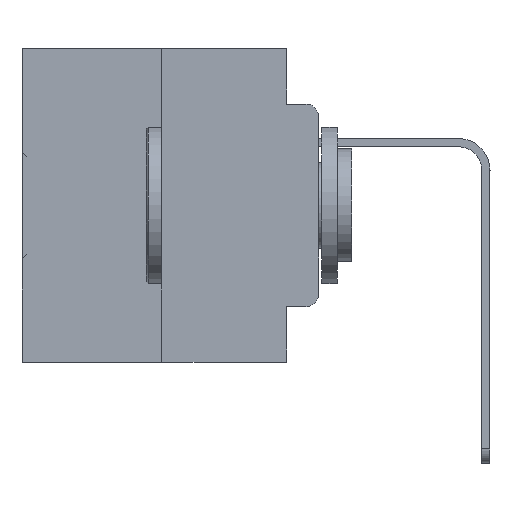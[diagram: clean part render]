
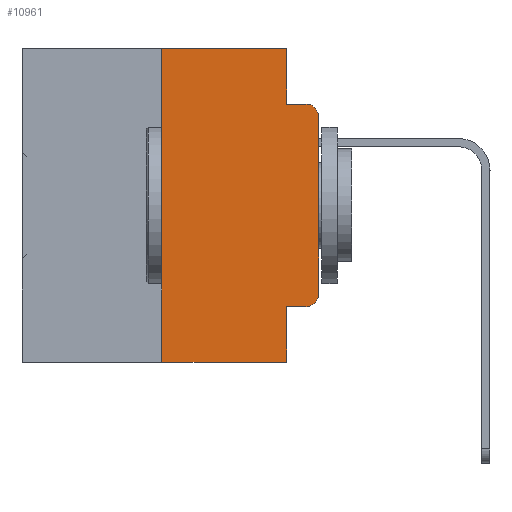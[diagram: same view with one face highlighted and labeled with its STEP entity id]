
A CAD part, left-side view. The second image highlights one B-rep face of the part: STEP entity #10961.
In plain terms, the highlighted planar face has unit normal (-1, 0, 0).
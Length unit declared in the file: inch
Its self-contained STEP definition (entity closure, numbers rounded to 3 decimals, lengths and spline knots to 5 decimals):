
#438 = VERTEX_POINT ( 'NONE', #14731 ) ;
#666 = CARTESIAN_POINT ( 'NONE',  ( 0., 0.051, 0. ) ) ;
#1281 = VERTEX_POINT ( 'NONE', #26488 ) ;
#1385 = CARTESIAN_POINT ( 'NONE',  ( 0., 0., -0.3915 ) ) ;
#1477 = ORIENTED_EDGE ( 'NONE', *, *, #6931, .F. ) ;
#1516 = CARTESIAN_POINT ( 'NONE',  ( 0., 0.473, 0. ) ) ;
#1558 = VERTEX_POINT ( 'NONE', #2695 ) ;
#1998 = DIRECTION ( 'NONE',  ( -1., 0., 0. ) ) ;
#2036 = EDGE_CURVE ( 'NONE', #438, #9720, #26792, .T. ) ;
#2336 = EDGE_CURVE ( 'NONE', #17228, #1281, #18663, .T. ) ;
#2695 = CARTESIAN_POINT ( 'NONE',  ( 0., 0.051, -0.5 ) ) ;
#2988 = CARTESIAN_POINT ( 'NONE',  ( 0., 0.25, 0. ) ) ;
#3020 = ORIENTED_EDGE ( 'NONE', *, *, #28326, .F. ) ;
#4269 = VECTOR ( 'NONE', #19569, 39.37008 ) ;
#4581 = DIRECTION ( 'NONE',  ( 0., 0., -1. ) ) ;
#4801 = EDGE_CURVE ( 'NONE', #17228, #1558, #6444, .T. ) ;
#4955 = VECTOR ( 'NONE', #26230, 39.37008 ) ;
#5456 = DIRECTION ( 'NONE',  ( 0., 0., -1. ) ) ;
#6444 = LINE ( 'NONE', #22230, #8445 ) ;
#6547 = VERTEX_POINT ( 'NONE', #15219 ) ;
#6931 = EDGE_CURVE ( 'NONE', #1281, #10455, #14763, .T. ) ;
#7218 = ORIENTED_EDGE ( 'NONE', *, *, #23450, .T. ) ;
#7374 = ORIENTED_EDGE ( 'NONE', *, *, #30153, .T. ) ;
#7673 = ORIENTED_EDGE ( 'NONE', *, *, #2336, .F. ) ;
#8445 = VECTOR ( 'NONE', #29581, 39.37008 ) ;
#9720 = VERTEX_POINT ( 'NONE', #1385 ) ;
#10299 = CARTESIAN_POINT ( 'NONE',  ( 0., 0.02, -0.1085 ) ) ;
#10408 = CARTESIAN_POINT ( 'NONE',  ( 0., 0.051, 0. ) ) ;
#10444 = PLANE ( 'NONE',  #31735 ) ;
#10455 = VERTEX_POINT ( 'NONE', #10408 ) ;
#10961 = ADVANCED_FACE ( 'NONE', ( #22563 ), #10444, .F. ) ;
#10979 = DIRECTION ( 'NONE',  ( 0., 0., -1. ) ) ;
#10987 = EDGE_LOOP ( 'NONE', ( #7218, #30588, #27500, #31379, #1477, #7673, #29914, #3020, #7374, #13615 ) ) ;
#11016 = CIRCLE ( 'NONE', #33447, 0.02 ) ;
#11518 = VECTOR ( 'NONE', #18947, 39.37008 ) ;
#12852 = LINE ( 'NONE', #666, #32626 ) ;
#12928 = DIRECTION ( 'NONE',  ( 1., 0., 0. ) ) ;
#13252 = VECTOR ( 'NONE', #22661, 39.37008 ) ;
#13615 = ORIENTED_EDGE ( 'NONE', *, *, #2036, .T. ) ;
#14002 = CARTESIAN_POINT ( 'NONE',  ( 0., 0.051, -0.4115 ) ) ;
#14731 = CARTESIAN_POINT ( 'NONE',  ( 0., 0.02, -0.4115 ) ) ;
#14763 = LINE ( 'NONE', #1516, #4269 ) ;
#15219 = CARTESIAN_POINT ( 'NONE',  ( 0., 0.051, -0.0885 ) ) ;
#15835 = CARTESIAN_POINT ( 'NONE',  ( 0., 0.473, 0. ) ) ;
#17043 = CARTESIAN_POINT ( 'NONE',  ( 0., 0.051, 0. ) ) ;
#17228 = VERTEX_POINT ( 'NONE', #21655 ) ;
#17439 = CARTESIAN_POINT ( 'NONE',  ( 0., 0.02, -0.3915 ) ) ;
#18663 = LINE ( 'NONE', #2988, #4955 ) ;
#18947 = DIRECTION ( 'NONE',  ( 0., -1., 0. ) ) ;
#19176 = EDGE_CURVE ( 'NONE', #6547, #24709, #20516, .T. ) ;
#19569 = DIRECTION ( 'NONE',  ( 0., -1., 0. ) ) ;
#20093 = CARTESIAN_POINT ( 'NONE',  ( 0., 0.051, -0.0885 ) ) ;
#20516 = LINE ( 'NONE', #20093, #13252 ) ;
#21281 = LINE ( 'NONE', #17043, #27351 ) ;
#21655 = CARTESIAN_POINT ( 'NONE',  ( 0., 0.25, -0.5 ) ) ;
#22230 = CARTESIAN_POINT ( 'NONE',  ( 0., 0.473, -0.5 ) ) ;
#22563 = FACE_OUTER_BOUND ( 'NONE', #10987, .T. ) ;
#22661 = DIRECTION ( 'NONE',  ( 0., -1., 0. ) ) ;
#23066 = EDGE_CURVE ( 'NONE', #25257, #24709, #11016, .T. ) ;
#23450 = EDGE_CURVE ( 'NONE', #9720, #25257, #29543, .T. ) ;
#24709 = VERTEX_POINT ( 'NONE', #25147 ) ;
#25147 = CARTESIAN_POINT ( 'NONE',  ( 0., 0.02, -0.0885 ) ) ;
#25257 = VERTEX_POINT ( 'NONE', #29521 ) ;
#25696 = AXIS2_PLACEMENT_3D ( 'NONE', #17439, #1998, #4581 ) ;
#26230 = DIRECTION ( 'NONE',  ( 0., 0., 1. ) ) ;
#26488 = CARTESIAN_POINT ( 'NONE',  ( 0., 0.25, 0. ) ) ;
#26792 = CIRCLE ( 'NONE', #25696, 0.02 ) ;
#27170 = CARTESIAN_POINT ( 'NONE',  ( 0., 0., 0. ) ) ;
#27351 = VECTOR ( 'NONE', #32636, 39.37008 ) ;
#27500 = ORIENTED_EDGE ( 'NONE', *, *, #19176, .F. ) ;
#28326 = EDGE_CURVE ( 'NONE', #31108, #1558, #12852, .T. ) ;
#29521 = CARTESIAN_POINT ( 'NONE',  ( 0., 0., -0.1085 ) ) ;
#29543 = LINE ( 'NONE', #27170, #32800 ) ;
#29581 = DIRECTION ( 'NONE',  ( 0., -1., 0. ) ) ;
#29914 = ORIENTED_EDGE ( 'NONE', *, *, #4801, .T. ) ;
#30153 = EDGE_CURVE ( 'NONE', #31108, #438, #32919, .T. ) ;
#30588 = ORIENTED_EDGE ( 'NONE', *, *, #23066, .T. ) ;
#30698 = DIRECTION ( 'NONE',  ( -1., 0., 0. ) ) ;
#31108 = VERTEX_POINT ( 'NONE', #32067 ) ;
#31245 = EDGE_CURVE ( 'NONE', #10455, #6547, #21281, .T. ) ;
#31379 = ORIENTED_EDGE ( 'NONE', *, *, #31245, .F. ) ;
#31735 = AXIS2_PLACEMENT_3D ( 'NONE', #15835, #12928, #5456 ) ;
#32067 = CARTESIAN_POINT ( 'NONE',  ( 0., 0.051, -0.4115 ) ) ;
#32363 = DIRECTION ( 'NONE',  ( 0., 0., 1. ) ) ;
#32626 = VECTOR ( 'NONE', #10979, 39.37008 ) ;
#32636 = DIRECTION ( 'NONE',  ( 0., 0., -1. ) ) ;
#32800 = VECTOR ( 'NONE', #32363, 39.37008 ) ;
#32919 = LINE ( 'NONE', #14002, #11518 ) ;
#33310 = DIRECTION ( 'NONE',  ( 0., 0., -1. ) ) ;
#33447 = AXIS2_PLACEMENT_3D ( 'NONE', #10299, #30698, #33310 ) ;
